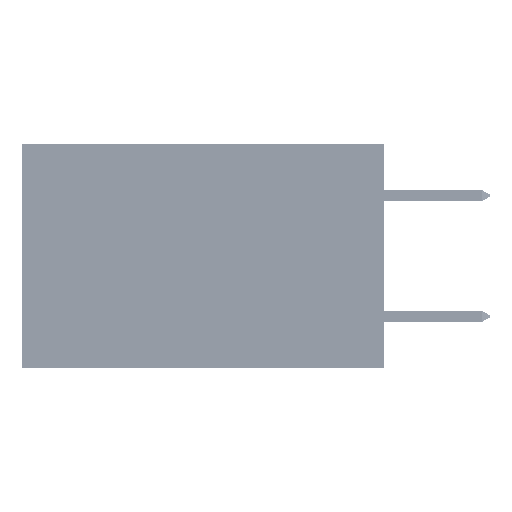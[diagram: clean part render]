
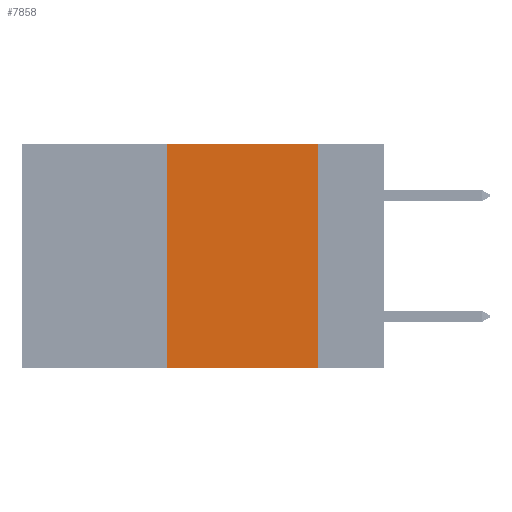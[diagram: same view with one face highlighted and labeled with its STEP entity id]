
A CAD part, left-side view. The second image highlights one B-rep face of the part: STEP entity #7858.
In plain terms, the highlighted planar face has unit normal (-1, 0, 0).
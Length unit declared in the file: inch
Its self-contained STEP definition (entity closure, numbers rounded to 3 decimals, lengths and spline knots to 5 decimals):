
#3617 = PLANE ( 'NONE',  #46223 ) ;
#4353 = CARTESIAN_POINT ( 'NONE',  ( 0., 0.36, 0. ) ) ;
#5901 = CARTESIAN_POINT ( 'NONE',  ( 0., 0.6, 0. ) ) ;
#7189 = CARTESIAN_POINT ( 'NONE',  ( 0., 0.6, 0. ) ) ;
#7858 = ADVANCED_FACE ( 'NONE', ( #13856 ), #3617, .F. ) ;
#9242 = LINE ( 'NONE', #4353, #31255 ) ;
#9849 = ORIENTED_EDGE ( 'NONE', *, *, #18895, .T. ) ;
#11731 = ORIENTED_EDGE ( 'NONE', *, *, #30385, .F. ) ;
#13522 = VECTOR ( 'NONE', #27787, 39.37008 ) ;
#13856 = FACE_OUTER_BOUND ( 'NONE', #23129, .T. ) ;
#16905 = VECTOR ( 'NONE', #17472, 39.37008 ) ;
#16918 = VERTEX_POINT ( 'NONE', #21182 ) ;
#17319 = CARTESIAN_POINT ( 'NONE',  ( 0., 0.11, 0. ) ) ;
#17472 = DIRECTION ( 'NONE',  ( 0., 0., -1. ) ) ;
#18152 = DIRECTION ( 'NONE',  ( 0., -1., 0. ) ) ;
#18756 = VERTEX_POINT ( 'NONE', #30745 ) ;
#18895 = EDGE_CURVE ( 'NONE', #16918, #18756, #36043, .T. ) ;
#19962 = DIRECTION ( 'NONE',  ( 0., 0., 1. ) ) ;
#21182 = CARTESIAN_POINT ( 'NONE',  ( 0., 0.36, -0.37 ) ) ;
#21408 = CARTESIAN_POINT ( 'NONE',  ( 0., 0.6, -0.37 ) ) ;
#22000 = DIRECTION ( 'NONE',  ( 1., 0., 0. ) ) ;
#23129 = EDGE_LOOP ( 'NONE', ( #11731, #33063, #44674, #9849 ) ) ;
#24908 = EDGE_CURVE ( 'NONE', #16918, #31001, #9242, .T. ) ;
#25492 = VECTOR ( 'NONE', #18152, 39.37008 ) ;
#25690 = DIRECTION ( 'NONE',  ( 0., 0., -1. ) ) ;
#26261 = VERTEX_POINT ( 'NONE', #34997 ) ;
#27787 = DIRECTION ( 'NONE',  ( 0., -1., 0. ) ) ;
#30385 = EDGE_CURVE ( 'NONE', #26261, #18756, #33041, .T. ) ;
#30745 = CARTESIAN_POINT ( 'NONE',  ( 0., 0.11, -0.37 ) ) ;
#31001 = VERTEX_POINT ( 'NONE', #47127 ) ;
#31255 = VECTOR ( 'NONE', #19962, 39.37008 ) ;
#33041 = LINE ( 'NONE', #17319, #16905 ) ;
#33063 = ORIENTED_EDGE ( 'NONE', *, *, #40658, .F. ) ;
#34997 = CARTESIAN_POINT ( 'NONE',  ( 0., 0.11, 0. ) ) ;
#36043 = LINE ( 'NONE', #21408, #25492 ) ;
#36047 = LINE ( 'NONE', #5901, #13522 ) ;
#40658 = EDGE_CURVE ( 'NONE', #31001, #26261, #36047, .T. ) ;
#44674 = ORIENTED_EDGE ( 'NONE', *, *, #24908, .F. ) ;
#46223 = AXIS2_PLACEMENT_3D ( 'NONE', #7189, #22000, #25690 ) ;
#47127 = CARTESIAN_POINT ( 'NONE',  ( 0., 0.36, 0. ) ) ;
